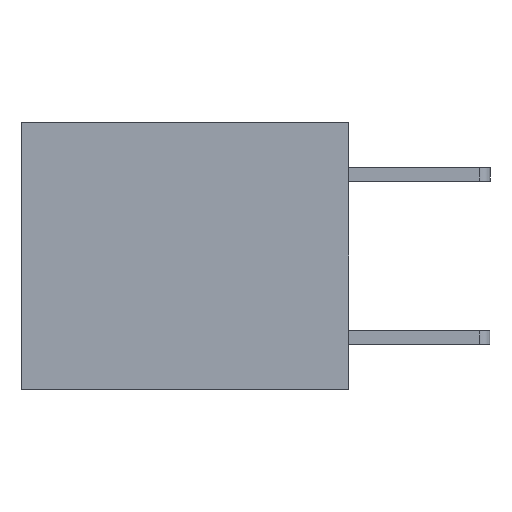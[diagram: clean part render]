
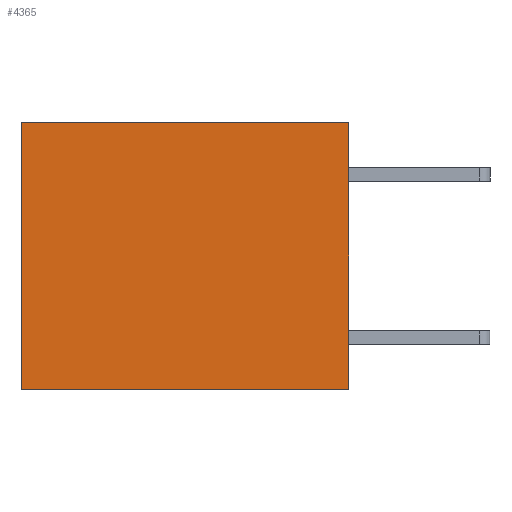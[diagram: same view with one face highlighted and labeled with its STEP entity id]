
A CAD part, left-side view. The second image highlights one B-rep face of the part: STEP entity #4365.
In plain terms, the highlighted planar face has unit normal (-1, 0, 0).
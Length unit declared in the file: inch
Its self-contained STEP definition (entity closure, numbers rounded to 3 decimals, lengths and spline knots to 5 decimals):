
#401 = DIRECTION ( 'NONE',  ( 0., 0., -1. ) ) ;
#488 = EDGE_CURVE ( 'NONE', #10184, #3998, #7044, .T. ) ;
#526 = CARTESIAN_POINT ( 'NONE',  ( 0.3165, 0., 0. ) ) ;
#541 = DIRECTION ( 'NONE',  ( 0., 0., -1. ) ) ;
#729 = EDGE_LOOP ( 'NONE', ( #4413, #6431, #3213, #4019 ) ) ;
#1091 = EDGE_CURVE ( 'NONE', #7260, #10184, #3319, .T. ) ;
#1190 = CARTESIAN_POINT ( 'NONE',  ( 0.3165, 0., -0.49 ) ) ;
#1334 = PLANE ( 'NONE',  #7593 ) ;
#3213 = ORIENTED_EDGE ( 'NONE', *, *, #3251, .F. ) ;
#3251 = EDGE_CURVE ( 'NONE', #7260, #9500, #6158, .T. ) ;
#3319 = LINE ( 'NONE', #7422, #4942 ) ;
#3489 = DIRECTION ( 'NONE',  ( 0., 0., -1. ) ) ;
#3998 = VERTEX_POINT ( 'NONE', #4497 ) ;
#4019 = ORIENTED_EDGE ( 'NONE', *, *, #1091, .T. ) ;
#4365 = ADVANCED_FACE ( 'NONE', ( #4788 ), #1334, .F. ) ;
#4413 = ORIENTED_EDGE ( 'NONE', *, *, #488, .T. ) ;
#4497 = CARTESIAN_POINT ( 'NONE',  ( 0.3165, 0.6, -0.49 ) ) ;
#4783 = VECTOR ( 'NONE', #5752, 39.37008 ) ;
#4788 = FACE_OUTER_BOUND ( 'NONE', #729, .T. ) ;
#4942 = VECTOR ( 'NONE', #6080, 39.37008 ) ;
#5032 = LINE ( 'NONE', #8165, #4783 ) ;
#5080 = VECTOR ( 'NONE', #3489, 39.37008 ) ;
#5319 = DIRECTION ( 'NONE',  ( 1., 0., 0. ) ) ;
#5460 = EDGE_CURVE ( 'NONE', #9500, #3998, #5032, .T. ) ;
#5752 = DIRECTION ( 'NONE',  ( 0., 1., 0. ) ) ;
#6080 = DIRECTION ( 'NONE',  ( 0., 1., 0. ) ) ;
#6158 = LINE ( 'NONE', #1190, #8027 ) ;
#6431 = ORIENTED_EDGE ( 'NONE', *, *, #5460, .F. ) ;
#7044 = LINE ( 'NONE', #9885, #5080 ) ;
#7260 = VERTEX_POINT ( 'NONE', #526 ) ;
#7422 = CARTESIAN_POINT ( 'NONE',  ( 0.3165, 0., 0. ) ) ;
#7593 = AXIS2_PLACEMENT_3D ( 'NONE', #10039, #5319, #541 ) ;
#8027 = VECTOR ( 'NONE', #401, 39.37008 ) ;
#8165 = CARTESIAN_POINT ( 'NONE',  ( 0.3165, 0., -0.49 ) ) ;
#9500 = VERTEX_POINT ( 'NONE', #9567 ) ;
#9567 = CARTESIAN_POINT ( 'NONE',  ( 0.3165, 0., -0.49 ) ) ;
#9885 = CARTESIAN_POINT ( 'NONE',  ( 0.3165, 0.6, -0.49 ) ) ;
#10007 = CARTESIAN_POINT ( 'NONE',  ( 0.3165, 0.6, 0. ) ) ;
#10039 = CARTESIAN_POINT ( 'NONE',  ( 0.3165, 0., -0.49 ) ) ;
#10184 = VERTEX_POINT ( 'NONE', #10007 ) ;
